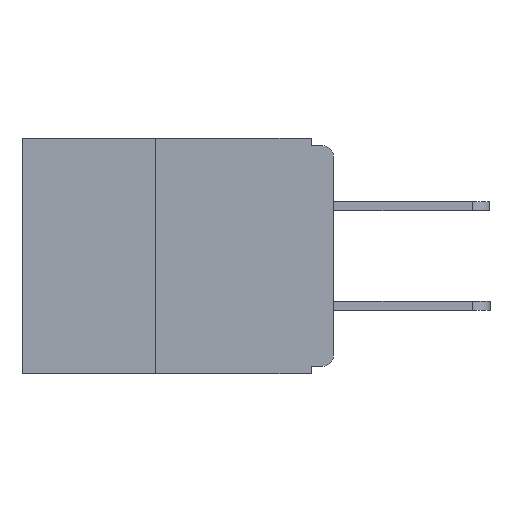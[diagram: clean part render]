
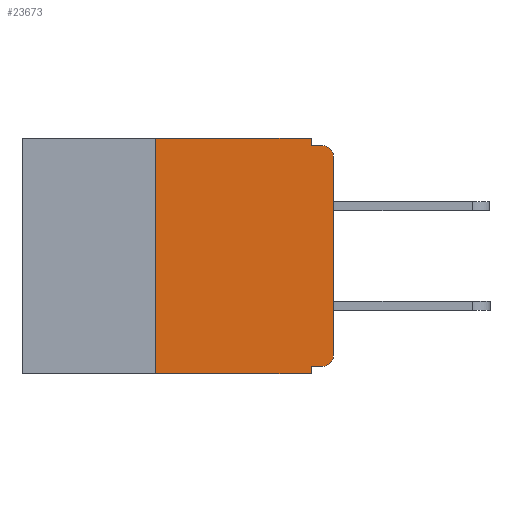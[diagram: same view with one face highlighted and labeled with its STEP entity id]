
A CAD part, left-side view. The second image highlights one B-rep face of the part: STEP entity #23673.
In plain terms, the highlighted planar face has unit normal (-1, 0, 0).
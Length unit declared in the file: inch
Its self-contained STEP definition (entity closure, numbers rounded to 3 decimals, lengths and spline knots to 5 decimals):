
#476 = DIRECTION ( 'NONE',  ( 0., 0., -1. ) ) ;
#1126 = DIRECTION ( 'NONE',  ( 0., 1., 0. ) ) ;
#1307 = CARTESIAN_POINT ( 'NONE',  ( 0., 0., 0. ) ) ;
#1588 = AXIS2_PLACEMENT_3D ( 'NONE', #3226, #3402, #18220 ) ;
#2040 = ORIENTED_EDGE ( 'NONE', *, *, #18262, .F. ) ;
#2311 = CARTESIAN_POINT ( 'NONE',  ( 0., 0.25, 0. ) ) ;
#2741 = CIRCLE ( 'NONE', #20188, 0.015 ) ;
#3094 = LINE ( 'NONE', #4928, #13747 ) ;
#3152 = ORIENTED_EDGE ( 'NONE', *, *, #18529, .F. ) ;
#3226 = CARTESIAN_POINT ( 'NONE',  ( 0., 0.437, 0. ) ) ;
#3402 = DIRECTION ( 'NONE',  ( 1., 0., 0. ) ) ;
#3734 = VECTOR ( 'NONE', #25146, 39.37008 ) ;
#3931 = EDGE_CURVE ( 'NONE', #9673, #20734, #26174, .T. ) ;
#4433 = LINE ( 'NONE', #12685, #3734 ) ;
#4928 = CARTESIAN_POINT ( 'NONE',  ( 0., 0., -0.01 ) ) ;
#5421 = VECTOR ( 'NONE', #9404, 39.37008 ) ;
#5425 = LINE ( 'NONE', #26309, #26960 ) ;
#5670 = DIRECTION ( 'NONE',  ( 0., -1., 0. ) ) ;
#6055 = DIRECTION ( 'NONE',  ( -1., 0., 0. ) ) ;
#7958 = ORIENTED_EDGE ( 'NONE', *, *, #20077, .T. ) ;
#8266 = CARTESIAN_POINT ( 'NONE',  ( 0., 0., -0.305 ) ) ;
#8290 = CARTESIAN_POINT ( 'NONE',  ( 0., 0.031, -0.32 ) ) ;
#8324 = VECTOR ( 'NONE', #5670, 39.37008 ) ;
#8333 = VECTOR ( 'NONE', #476, 39.37008 ) ;
#8819 = ORIENTED_EDGE ( 'NONE', *, *, #17599, .F. ) ;
#9037 = ORIENTED_EDGE ( 'NONE', *, *, #22315, .F. ) ;
#9404 = DIRECTION ( 'NONE',  ( 0., 0., 1. ) ) ;
#9673 = VERTEX_POINT ( 'NONE', #26834 ) ;
#9678 = VERTEX_POINT ( 'NONE', #18715 ) ;
#10051 = CARTESIAN_POINT ( 'NONE',  ( 0., 0.031, -0.33 ) ) ;
#10341 = VECTOR ( 'NONE', #14146, 39.37008 ) ;
#10773 = CARTESIAN_POINT ( 'NONE',  ( 0., 0.031, -0.33 ) ) ;
#11771 = LINE ( 'NONE', #13615, #5421 ) ;
#12324 = CARTESIAN_POINT ( 'NONE',  ( 0., 0.015, -0.025 ) ) ;
#12382 = FACE_OUTER_BOUND ( 'NONE', #16060, .T. ) ;
#12685 = CARTESIAN_POINT ( 'NONE',  ( 0., 0.437, 0. ) ) ;
#13271 = EDGE_CURVE ( 'NONE', #20734, #17613, #20871, .T. ) ;
#13615 = CARTESIAN_POINT ( 'NONE',  ( 0., 0.25, -0.33 ) ) ;
#13747 = VECTOR ( 'NONE', #23830, 39.37008 ) ;
#14146 = DIRECTION ( 'NONE',  ( 0., 0., 1. ) ) ;
#14197 = CARTESIAN_POINT ( 'NONE',  ( 0., 0.031, -0.01 ) ) ;
#14415 = DIRECTION ( 'NONE',  ( 0., 0., -1. ) ) ;
#14629 = LINE ( 'NONE', #18254, #8324 ) ;
#14923 = VERTEX_POINT ( 'NONE', #2311 ) ;
#15450 = CARTESIAN_POINT ( 'NONE',  ( 0., 0.031, 0. ) ) ;
#15890 = AXIS2_PLACEMENT_3D ( 'NONE', #18721, #6055, #20839 ) ;
#16060 = EDGE_LOOP ( 'NONE', ( #17609, #18086, #9037, #23277, #3152, #8819, #7958, #21059, #2040, #24153 ) ) ;
#16087 = VERTEX_POINT ( 'NONE', #10773 ) ;
#16190 = CARTESIAN_POINT ( 'NONE',  ( 0., 0.015, -0.01 ) ) ;
#16662 = VERTEX_POINT ( 'NONE', #19109 ) ;
#17145 = VERTEX_POINT ( 'NONE', #14197 ) ;
#17599 = EDGE_CURVE ( 'NONE', #9678, #14923, #11771, .T. ) ;
#17609 = ORIENTED_EDGE ( 'NONE', *, *, #13271, .T. ) ;
#17613 = VERTEX_POINT ( 'NONE', #26062 ) ;
#18086 = ORIENTED_EDGE ( 'NONE', *, *, #18402, .T. ) ;
#18220 = DIRECTION ( 'NONE',  ( 0., 0., -1. ) ) ;
#18254 = CARTESIAN_POINT ( 'NONE',  ( 0., 0.437, -0.33 ) ) ;
#18262 = EDGE_CURVE ( 'NONE', #9673, #18524, #5425, .T. ) ;
#18402 = EDGE_CURVE ( 'NONE', #17613, #23722, #2741, .T. ) ;
#18524 = VERTEX_POINT ( 'NONE', #8290 ) ;
#18529 = EDGE_CURVE ( 'NONE', #14923, #16662, #4433, .T. ) ;
#18534 = DIRECTION ( 'NONE',  ( 0., 0., -1. ) ) ;
#18715 = CARTESIAN_POINT ( 'NONE',  ( 0., 0.25, -0.33 ) ) ;
#18721 = CARTESIAN_POINT ( 'NONE',  ( 0., 0.015, -0.305 ) ) ;
#18890 = VECTOR ( 'NONE', #18534, 39.37008 ) ;
#19109 = CARTESIAN_POINT ( 'NONE',  ( 0., 0.031, 0. ) ) ;
#19536 = LINE ( 'NONE', #10051, #18890 ) ;
#19541 = LINE ( 'NONE', #15450, #8333 ) ;
#20077 = EDGE_CURVE ( 'NONE', #9678, #16087, #14629, .T. ) ;
#20115 = EDGE_CURVE ( 'NONE', #18524, #16087, #19536, .T. ) ;
#20188 = AXIS2_PLACEMENT_3D ( 'NONE', #12324, #26739, #14415 ) ;
#20734 = VERTEX_POINT ( 'NONE', #8266 ) ;
#20839 = DIRECTION ( 'NONE',  ( 0., 0., -1. ) ) ;
#20871 = LINE ( 'NONE', #1307, #10341 ) ;
#21059 = ORIENTED_EDGE ( 'NONE', *, *, #20115, .F. ) ;
#22315 = EDGE_CURVE ( 'NONE', #17145, #23722, #3094, .T. ) ;
#23277 = ORIENTED_EDGE ( 'NONE', *, *, #27155, .F. ) ;
#23673 = ADVANCED_FACE ( 'NONE', ( #12382 ), #24341, .F. ) ;
#23722 = VERTEX_POINT ( 'NONE', #16190 ) ;
#23830 = DIRECTION ( 'NONE',  ( 0., -1., 0. ) ) ;
#24153 = ORIENTED_EDGE ( 'NONE', *, *, #3931, .T. ) ;
#24341 = PLANE ( 'NONE',  #1588 ) ;
#25146 = DIRECTION ( 'NONE',  ( 0., -1., 0. ) ) ;
#26062 = CARTESIAN_POINT ( 'NONE',  ( 0., 0., -0.025 ) ) ;
#26174 = CIRCLE ( 'NONE', #15890, 0.015 ) ;
#26309 = CARTESIAN_POINT ( 'NONE',  ( 0., 0., -0.32 ) ) ;
#26739 = DIRECTION ( 'NONE',  ( -1., 0., 0. ) ) ;
#26834 = CARTESIAN_POINT ( 'NONE',  ( 0., 0.015, -0.32 ) ) ;
#26960 = VECTOR ( 'NONE', #1126, 39.37008 ) ;
#27155 = EDGE_CURVE ( 'NONE', #16662, #17145, #19541, .T. ) ;
